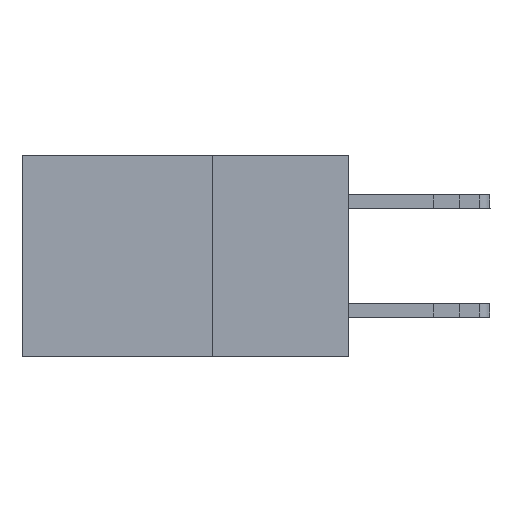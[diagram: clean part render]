
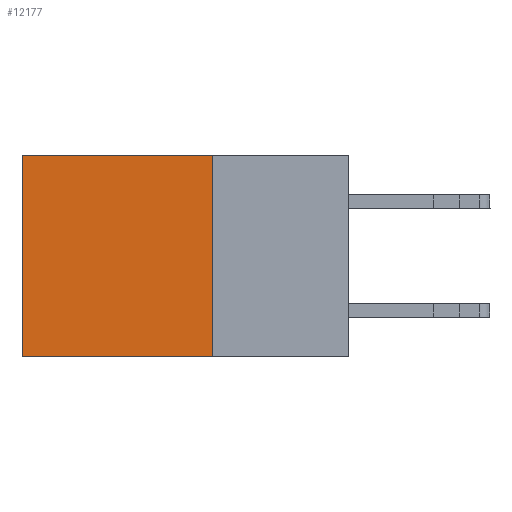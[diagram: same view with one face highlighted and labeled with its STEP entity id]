
A CAD part, left-side view. The second image highlights one B-rep face of the part: STEP entity #12177.
In plain terms, the highlighted planar face has unit normal (-1, 0, 0).
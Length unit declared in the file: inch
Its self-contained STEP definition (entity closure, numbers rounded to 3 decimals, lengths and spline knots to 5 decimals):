
#458 = CARTESIAN_POINT ( 'NONE',  ( 0.2615, 0.25, 0. ) ) ;
#516 = ORIENTED_EDGE ( 'NONE', *, *, #8576, .T. ) ;
#947 = EDGE_LOOP ( 'NONE', ( #11434, #14724, #4017, #516 ) ) ;
#1334 = CARTESIAN_POINT ( 'NONE',  ( 0.2615, 0.6, -0.37 ) ) ;
#1423 = LINE ( 'NONE', #9475, #10201 ) ;
#1434 = PLANE ( 'NONE',  #7559 ) ;
#2589 = CARTESIAN_POINT ( 'NONE',  ( 0.2615, 0.6, 0. ) ) ;
#4017 = ORIENTED_EDGE ( 'NONE', *, *, #8802, .F. ) ;
#4158 = DIRECTION ( 'NONE',  ( 0., 0., -1. ) ) ;
#4266 = DIRECTION ( 'NONE',  ( 0., 1., 0. ) ) ;
#4660 = CARTESIAN_POINT ( 'NONE',  ( 0.2615, 0.25, -0.37 ) ) ;
#5829 = CARTESIAN_POINT ( 'NONE',  ( 0.2615, 0.6, -0.37 ) ) ;
#6074 = CARTESIAN_POINT ( 'NONE',  ( 0.2615, 0.25, -0.37 ) ) ;
#7559 = AXIS2_PLACEMENT_3D ( 'NONE', #14302, #12517, #4158 ) ;
#7972 = CARTESIAN_POINT ( 'NONE',  ( 0.2615, 0.25, -0.37 ) ) ;
#8430 = VERTEX_POINT ( 'NONE', #5829 ) ;
#8576 = EDGE_CURVE ( 'NONE', #19589, #10775, #1423, .T. ) ;
#8802 = EDGE_CURVE ( 'NONE', #19589, #15756, #20531, .T. ) ;
#9475 = CARTESIAN_POINT ( 'NONE',  ( 0.2615, 0.25, 0. ) ) ;
#9486 = FACE_OUTER_BOUND ( 'NONE', #947, .T. ) ;
#9546 = EDGE_CURVE ( 'NONE', #15756, #8430, #18989, .T. ) ;
#10201 = VECTOR ( 'NONE', #4266, 39.37008 ) ;
#10775 = VERTEX_POINT ( 'NONE', #2589 ) ;
#10833 = DIRECTION ( 'NONE',  ( 0., 1., 0. ) ) ;
#11434 = ORIENTED_EDGE ( 'NONE', *, *, #13529, .T. ) ;
#12177 = ADVANCED_FACE ( 'NONE', ( #9486 ), #1434, .F. ) ;
#12517 = DIRECTION ( 'NONE',  ( 1., 0., 0. ) ) ;
#13134 = VECTOR ( 'NONE', #10833, 39.37008 ) ;
#13529 = EDGE_CURVE ( 'NONE', #10775, #8430, #15766, .T. ) ;
#14302 = CARTESIAN_POINT ( 'NONE',  ( 0.2615, 0.25, -0.37 ) ) ;
#14724 = ORIENTED_EDGE ( 'NONE', *, *, #9546, .F. ) ;
#15756 = VERTEX_POINT ( 'NONE', #4660 ) ;
#15766 = LINE ( 'NONE', #1334, #16004 ) ;
#16004 = VECTOR ( 'NONE', #17550, 39.37008 ) ;
#17550 = DIRECTION ( 'NONE',  ( 0., 0., -1. ) ) ;
#18989 = LINE ( 'NONE', #7972, #13134 ) ;
#19044 = DIRECTION ( 'NONE',  ( 0., 0., -1. ) ) ;
#19559 = VECTOR ( 'NONE', #19044, 39.37008 ) ;
#19589 = VERTEX_POINT ( 'NONE', #458 ) ;
#20531 = LINE ( 'NONE', #6074, #19559 ) ;
